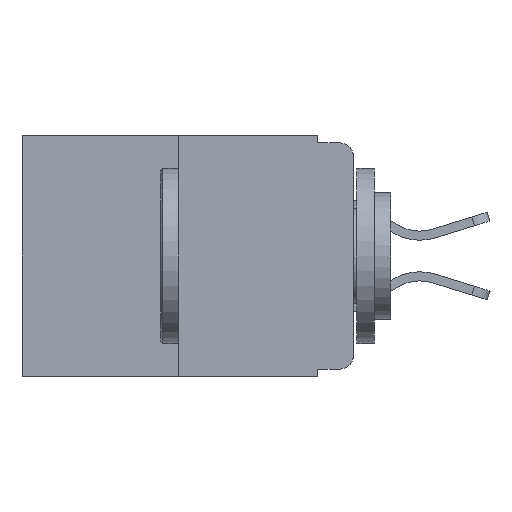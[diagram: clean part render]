
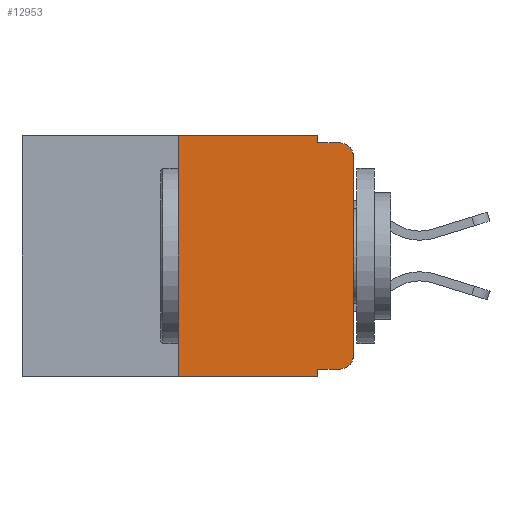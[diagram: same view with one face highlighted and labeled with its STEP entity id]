
A CAD part, left-side view. The second image highlights one B-rep face of the part: STEP entity #12953.
In plain terms, the highlighted planar face has unit normal (-1, 0, 0).
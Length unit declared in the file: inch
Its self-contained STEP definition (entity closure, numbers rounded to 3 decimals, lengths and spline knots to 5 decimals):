
#4 = CARTESIAN_POINT ( 'NONE',  ( 0., 0.051, -0.333 ) ) ;
#162 = DIRECTION ( 'NONE',  ( 0., 0., -1. ) ) ;
#294 = CARTESIAN_POINT ( 'NONE',  ( 0., 0., -0.03 ) ) ;
#300 = DIRECTION ( 'NONE',  ( -1., 0., 0. ) ) ;
#315 = VERTEX_POINT ( 'NONE', #4924 ) ;
#1033 = LINE ( 'NONE', #4, #2411 ) ;
#1080 = EDGE_CURVE ( 'NONE', #14466, #4872, #12206, .T. ) ;
#1146 = CARTESIAN_POINT ( 'NONE',  ( 0., 0.051, -0.343 ) ) ;
#1360 = CARTESIAN_POINT ( 'NONE',  ( 0., 0.473, 0. ) ) ;
#1461 = AXIS2_PLACEMENT_3D ( 'NONE', #12581, #12656, #4667 ) ;
#1471 = CARTESIAN_POINT ( 'NONE',  ( 0., 0.051, -0.333 ) ) ;
#1797 = VECTOR ( 'NONE', #7034, 39.37008 ) ;
#2411 = VECTOR ( 'NONE', #6570, 39.37008 ) ;
#2635 = PLANE ( 'NONE',  #9988 ) ;
#3523 = LINE ( 'NONE', #3673, #1797 ) ;
#3541 = CARTESIAN_POINT ( 'NONE',  ( 0., 0.473, -0.343 ) ) ;
#3607 = LINE ( 'NONE', #14690, #12778 ) ;
#3673 = CARTESIAN_POINT ( 'NONE',  ( 0., 0.051, -0.01 ) ) ;
#3687 = EDGE_CURVE ( 'NONE', #315, #13967, #5186, .T. ) ;
#3688 = DIRECTION ( 'NONE',  ( 0., -1., 0. ) ) ;
#3709 = VECTOR ( 'NONE', #4152, 39.37008 ) ;
#4011 = VECTOR ( 'NONE', #4737, 39.37008 ) ;
#4152 = DIRECTION ( 'NONE',  ( 0., 0., 1. ) ) ;
#4335 = VERTEX_POINT ( 'NONE', #6965 ) ;
#4372 = CARTESIAN_POINT ( 'NONE',  ( 0., 0.25, 0. ) ) ;
#4373 = EDGE_CURVE ( 'NONE', #5480, #4872, #3523, .T. ) ;
#4483 = ORIENTED_EDGE ( 'NONE', *, *, #5669, .T. ) ;
#4592 = DIRECTION ( 'NONE',  ( 0., 0., -1. ) ) ;
#4667 = DIRECTION ( 'NONE',  ( 0., 0., -1. ) ) ;
#4737 = DIRECTION ( 'NONE',  ( 0., -1., 0. ) ) ;
#4869 = DIRECTION ( 'NONE',  ( 0., 0., -1. ) ) ;
#4872 = VERTEX_POINT ( 'NONE', #10760 ) ;
#4924 = CARTESIAN_POINT ( 'NONE',  ( 0., 0.25, -0.343 ) ) ;
#5186 = LINE ( 'NONE', #7432, #3709 ) ;
#5384 = ORIENTED_EDGE ( 'NONE', *, *, #14054, .F. ) ;
#5480 = VERTEX_POINT ( 'NONE', #13637 ) ;
#5556 = ORIENTED_EDGE ( 'NONE', *, *, #14134, .T. ) ;
#5610 = VECTOR ( 'NONE', #162, 39.37008 ) ;
#5669 = EDGE_CURVE ( 'NONE', #11694, #4335, #6627, .T. ) ;
#5693 = AXIS2_PLACEMENT_3D ( 'NONE', #10409, #300, #4869 ) ;
#5863 = LINE ( 'NONE', #1360, #11169 ) ;
#5896 = EDGE_CURVE ( 'NONE', #10580, #11694, #1033, .T. ) ;
#6570 = DIRECTION ( 'NONE',  ( 0., -1., 0. ) ) ;
#6627 = CIRCLE ( 'NONE', #5693, 0.02 ) ;
#6848 = CARTESIAN_POINT ( 'NONE',  ( 0., 0., 0. ) ) ;
#6929 = ORIENTED_EDGE ( 'NONE', *, *, #3687, .F. ) ;
#6939 = VERTEX_POINT ( 'NONE', #1146 ) ;
#6965 = CARTESIAN_POINT ( 'NONE',  ( 0., 0., -0.313 ) ) ;
#6968 = VERTEX_POINT ( 'NONE', #7130 ) ;
#6972 = LINE ( 'NONE', #9070, #5610 ) ;
#7034 = DIRECTION ( 'NONE',  ( 0., -1., 0. ) ) ;
#7068 = ORIENTED_EDGE ( 'NONE', *, *, #7619, .T. ) ;
#7111 = ORIENTED_EDGE ( 'NONE', *, *, #8244, .F. ) ;
#7130 = CARTESIAN_POINT ( 'NONE',  ( 0., 0.051, 0. ) ) ;
#7432 = CARTESIAN_POINT ( 'NONE',  ( 0., 0.25, 0. ) ) ;
#7606 = DIRECTION ( 'NONE',  ( 0., 0., -1. ) ) ;
#7619 = EDGE_CURVE ( 'NONE', #4335, #14466, #12430, .T. ) ;
#7684 = DIRECTION ( 'NONE',  ( 1., 0., 0. ) ) ;
#8244 = EDGE_CURVE ( 'NONE', #6968, #5480, #3607, .T. ) ;
#8624 = VECTOR ( 'NONE', #11412, 39.37008 ) ;
#8807 = FACE_OUTER_BOUND ( 'NONE', #11266, .T. ) ;
#9070 = CARTESIAN_POINT ( 'NONE',  ( 0., 0.051, 0. ) ) ;
#9460 = EDGE_CURVE ( 'NONE', #10580, #6939, #6972, .T. ) ;
#9988 = AXIS2_PLACEMENT_3D ( 'NONE', #12880, #7684, #7606 ) ;
#10409 = CARTESIAN_POINT ( 'NONE',  ( 0., 0.02, -0.313 ) ) ;
#10571 = LINE ( 'NONE', #3541, #4011 ) ;
#10580 = VERTEX_POINT ( 'NONE', #1471 ) ;
#10639 = ORIENTED_EDGE ( 'NONE', *, *, #9460, .F. ) ;
#10760 = CARTESIAN_POINT ( 'NONE',  ( 0., 0.02, -0.01 ) ) ;
#10769 = ORIENTED_EDGE ( 'NONE', *, *, #5896, .T. ) ;
#11169 = VECTOR ( 'NONE', #3688, 39.37008 ) ;
#11266 = EDGE_LOOP ( 'NONE', ( #7068, #13168, #13212, #7111, #5384, #6929, #5556, #10639, #10769, #4483 ) ) ;
#11412 = DIRECTION ( 'NONE',  ( 0., 0., 1. ) ) ;
#11694 = VERTEX_POINT ( 'NONE', #14585 ) ;
#12206 = CIRCLE ( 'NONE', #1461, 0.02 ) ;
#12430 = LINE ( 'NONE', #6848, #8624 ) ;
#12581 = CARTESIAN_POINT ( 'NONE',  ( 0., 0.02, -0.03 ) ) ;
#12656 = DIRECTION ( 'NONE',  ( -1., 0., 0. ) ) ;
#12778 = VECTOR ( 'NONE', #4592, 39.37008 ) ;
#12880 = CARTESIAN_POINT ( 'NONE',  ( 0., 0.473, 0. ) ) ;
#12953 = ADVANCED_FACE ( 'NONE', ( #8807 ), #2635, .F. ) ;
#13168 = ORIENTED_EDGE ( 'NONE', *, *, #1080, .T. ) ;
#13212 = ORIENTED_EDGE ( 'NONE', *, *, #4373, .F. ) ;
#13637 = CARTESIAN_POINT ( 'NONE',  ( 0., 0.051, -0.01 ) ) ;
#13967 = VERTEX_POINT ( 'NONE', #4372 ) ;
#14054 = EDGE_CURVE ( 'NONE', #13967, #6968, #5863, .T. ) ;
#14134 = EDGE_CURVE ( 'NONE', #315, #6939, #10571, .T. ) ;
#14466 = VERTEX_POINT ( 'NONE', #294 ) ;
#14585 = CARTESIAN_POINT ( 'NONE',  ( 0., 0.02, -0.333 ) ) ;
#14690 = CARTESIAN_POINT ( 'NONE',  ( 0., 0.051, 0. ) ) ;
